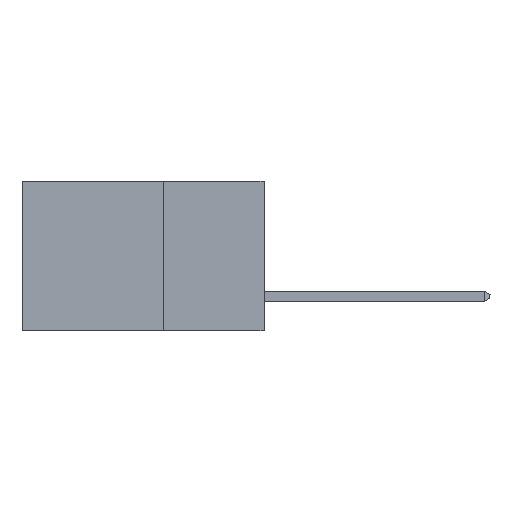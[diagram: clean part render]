
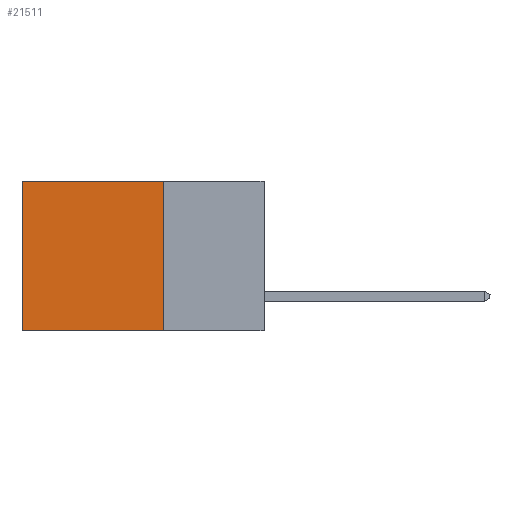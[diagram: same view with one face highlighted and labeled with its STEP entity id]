
A CAD part, left-side view. The second image highlights one B-rep face of the part: STEP entity #21511.
In plain terms, the highlighted planar face has unit normal (-1, 0, 0).
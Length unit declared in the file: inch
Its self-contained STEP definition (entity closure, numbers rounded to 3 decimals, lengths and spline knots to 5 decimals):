
#1391 = VERTEX_POINT ( 'NONE', #9743 ) ;
#1961 = EDGE_LOOP ( 'NONE', ( #31888, #27218, #12574, #4856 ) ) ;
#4200 = LINE ( 'NONE', #26936, #29333 ) ;
#4856 = ORIENTED_EDGE ( 'NONE', *, *, #25789, .T. ) ;
#6548 = AXIS2_PLACEMENT_3D ( 'NONE', #8749, #11624, #31715 ) ;
#8749 = CARTESIAN_POINT ( 'NONE',  ( 0.298, 0.25, 0. ) ) ;
#8892 = DIRECTION ( 'NONE',  ( 0., 0., -1. ) ) ;
#9039 = VECTOR ( 'NONE', #22247, 39.37008 ) ;
#9180 = CARTESIAN_POINT ( 'NONE',  ( 0.298, 0.25, -0.37 ) ) ;
#9298 = CARTESIAN_POINT ( 'NONE',  ( 0.298, 0.25, 0. ) ) ;
#9743 = CARTESIAN_POINT ( 'NONE',  ( 0.298, 0.6, -0.37 ) ) ;
#10022 = CARTESIAN_POINT ( 'NONE',  ( 0.298, 0.25, 0. ) ) ;
#10809 = VERTEX_POINT ( 'NONE', #30858 ) ;
#11016 = VERTEX_POINT ( 'NONE', #9298 ) ;
#11624 = DIRECTION ( 'NONE',  ( 1., 0., 0. ) ) ;
#11633 = DIRECTION ( 'NONE',  ( 0., 1., 0. ) ) ;
#12574 = ORIENTED_EDGE ( 'NONE', *, *, #15638, .F. ) ;
#13654 = CARTESIAN_POINT ( 'NONE',  ( 0.298, 0.6, 0. ) ) ;
#14686 = VECTOR ( 'NONE', #25207, 39.37008 ) ;
#15366 = LINE ( 'NONE', #13654, #28180 ) ;
#15480 = LINE ( 'NONE', #10022, #14686 ) ;
#15638 = EDGE_CURVE ( 'NONE', #11016, #10809, #15480, .T. ) ;
#17229 = CARTESIAN_POINT ( 'NONE',  ( 0.298, 0.6, 0. ) ) ;
#19112 = FACE_OUTER_BOUND ( 'NONE', #1961, .T. ) ;
#21511 = ADVANCED_FACE ( 'NONE', ( #19112 ), #31926, .F. ) ;
#22247 = DIRECTION ( 'NONE',  ( 0., 1., 0. ) ) ;
#23538 = EDGE_CURVE ( 'NONE', #29855, #1391, #15366, .T. ) ;
#23840 = LINE ( 'NONE', #9180, #9039 ) ;
#25207 = DIRECTION ( 'NONE',  ( 0., 0., -1. ) ) ;
#25789 = EDGE_CURVE ( 'NONE', #11016, #29855, #4200, .T. ) ;
#26936 = CARTESIAN_POINT ( 'NONE',  ( 0.298, 0.25, 0. ) ) ;
#27218 = ORIENTED_EDGE ( 'NONE', *, *, #32940, .F. ) ;
#28180 = VECTOR ( 'NONE', #8892, 39.37008 ) ;
#29333 = VECTOR ( 'NONE', #11633, 39.37008 ) ;
#29855 = VERTEX_POINT ( 'NONE', #17229 ) ;
#30858 = CARTESIAN_POINT ( 'NONE',  ( 0.298, 0.25, -0.37 ) ) ;
#31715 = DIRECTION ( 'NONE',  ( 0., 0., -1. ) ) ;
#31888 = ORIENTED_EDGE ( 'NONE', *, *, #23538, .T. ) ;
#31926 = PLANE ( 'NONE',  #6548 ) ;
#32940 = EDGE_CURVE ( 'NONE', #10809, #1391, #23840, .T. ) ;
